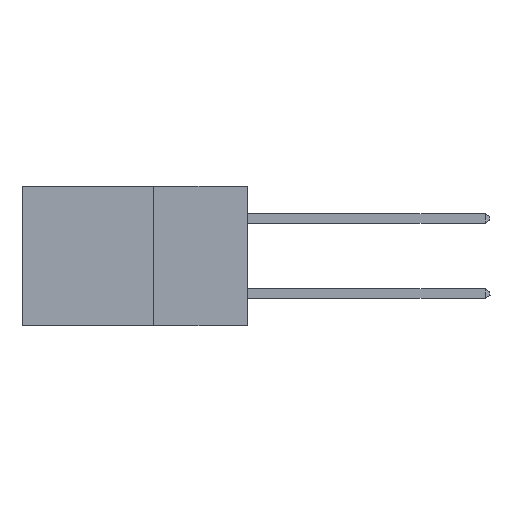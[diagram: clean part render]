
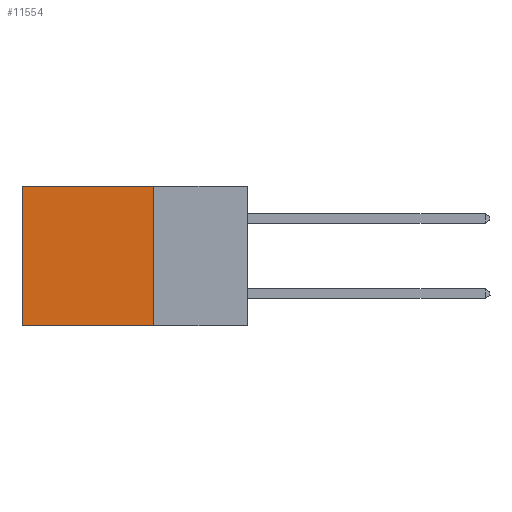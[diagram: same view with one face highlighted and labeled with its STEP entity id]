
A CAD part, left-side view. The second image highlights one B-rep face of the part: STEP entity #11554.
In plain terms, the highlighted planar face has unit normal (-1, 0, 0).
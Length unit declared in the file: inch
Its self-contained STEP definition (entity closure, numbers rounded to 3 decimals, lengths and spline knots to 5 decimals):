
#103 = PLANE ( 'NONE',  #1670 ) ;
#252 = DIRECTION ( 'NONE',  ( 0., 0., -1. ) ) ;
#279 = VECTOR ( 'NONE', #252, 39.37008 ) ;
#789 = FACE_OUTER_BOUND ( 'NONE', #7237, .T. ) ;
#839 = VECTOR ( 'NONE', #15834, 39.37008 ) ;
#923 = EDGE_CURVE ( 'NONE', #17002, #16073, #10473, .T. ) ;
#1670 = AXIS2_PLACEMENT_3D ( 'NONE', #7124, #13816, #20824 ) ;
#1788 = EDGE_CURVE ( 'NONE', #18027, #2757, #13421, .T. ) ;
#1827 = CARTESIAN_POINT ( 'NONE',  ( 0.298, 0.25, 0. ) ) ;
#2427 = ORIENTED_EDGE ( 'NONE', *, *, #18728, .F. ) ;
#2757 = VERTEX_POINT ( 'NONE', #2777 ) ;
#2777 = CARTESIAN_POINT ( 'NONE',  ( 0.298, 0.6, -0.37 ) ) ;
#2905 = VECTOR ( 'NONE', #3702, 39.37008 ) ;
#3702 = DIRECTION ( 'NONE',  ( 0., 0., -1. ) ) ;
#7124 = CARTESIAN_POINT ( 'NONE',  ( 0.298, 0.25, 0. ) ) ;
#7237 = EDGE_LOOP ( 'NONE', ( #14315, #14758, #2427, #20379 ) ) ;
#8025 = CARTESIAN_POINT ( 'NONE',  ( 0.298, 0.25, 0. ) ) ;
#10473 = LINE ( 'NONE', #1827, #839 ) ;
#11554 = ADVANCED_FACE ( 'NONE', ( #789 ), #103, .F. ) ;
#11782 = CARTESIAN_POINT ( 'NONE',  ( 0.298, 0.25, -0.37 ) ) ;
#13421 = LINE ( 'NONE', #11782, #20664 ) ;
#13816 = DIRECTION ( 'NONE',  ( 1., 0., 0. ) ) ;
#14256 = CARTESIAN_POINT ( 'NONE',  ( 0.298, 0.6, 0. ) ) ;
#14315 = ORIENTED_EDGE ( 'NONE', *, *, #21292, .T. ) ;
#14758 = ORIENTED_EDGE ( 'NONE', *, *, #1788, .F. ) ;
#15762 = CARTESIAN_POINT ( 'NONE',  ( 0.298, 0.25, 0. ) ) ;
#15834 = DIRECTION ( 'NONE',  ( 0., 1., 0. ) ) ;
#16073 = VERTEX_POINT ( 'NONE', #14256 ) ;
#17002 = VERTEX_POINT ( 'NONE', #8025 ) ;
#17435 = LINE ( 'NONE', #17500, #279 ) ;
#17500 = CARTESIAN_POINT ( 'NONE',  ( 0.298, 0.6, 0. ) ) ;
#18027 = VERTEX_POINT ( 'NONE', #21553 ) ;
#18728 = EDGE_CURVE ( 'NONE', #17002, #18027, #20346, .T. ) ;
#18843 = DIRECTION ( 'NONE',  ( 0., 1., 0. ) ) ;
#20346 = LINE ( 'NONE', #15762, #2905 ) ;
#20379 = ORIENTED_EDGE ( 'NONE', *, *, #923, .T. ) ;
#20664 = VECTOR ( 'NONE', #18843, 39.37008 ) ;
#20824 = DIRECTION ( 'NONE',  ( 0., 0., -1. ) ) ;
#21292 = EDGE_CURVE ( 'NONE', #16073, #2757, #17435, .T. ) ;
#21553 = CARTESIAN_POINT ( 'NONE',  ( 0.298, 0.25, -0.37 ) ) ;
